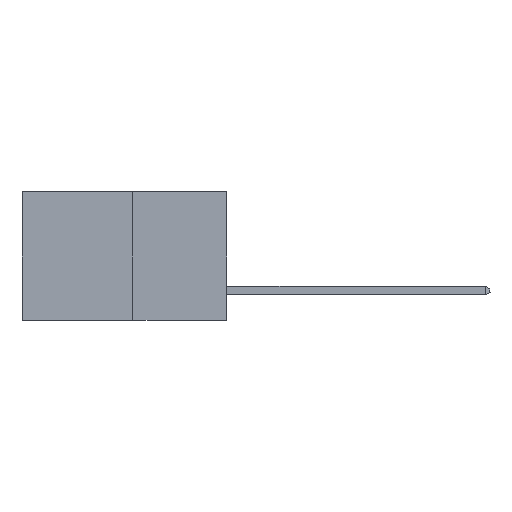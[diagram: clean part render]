
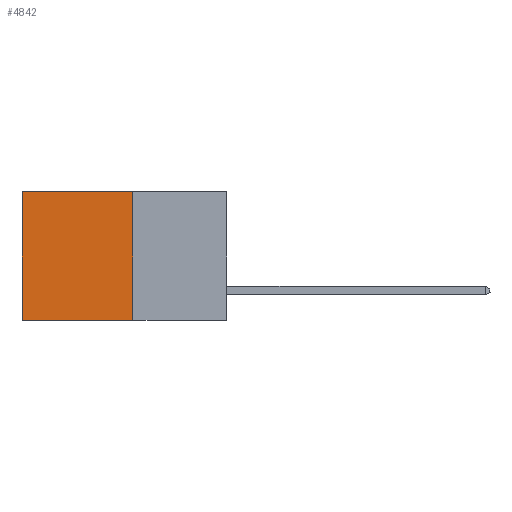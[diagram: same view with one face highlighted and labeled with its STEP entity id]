
A CAD part, left-side view. The second image highlights one B-rep face of the part: STEP entity #4842.
In plain terms, the highlighted planar face has unit normal (-1, 0, 0).
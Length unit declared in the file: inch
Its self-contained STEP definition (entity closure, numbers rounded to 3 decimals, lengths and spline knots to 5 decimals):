
#202 = CARTESIAN_POINT ( 'NONE',  ( 0.277, 0.27, -0.37 ) ) ;
#828 = ORIENTED_EDGE ( 'NONE', *, *, #5445, .F. ) ;
#1457 = DIRECTION ( 'NONE',  ( 1., 0., 0. ) ) ;
#1484 = LINE ( 'NONE', #5048, #11333 ) ;
#2099 = CARTESIAN_POINT ( 'NONE',  ( 0.277, 0.59, -0.37 ) ) ;
#2106 = DIRECTION ( 'NONE',  ( 0., 0., -1. ) ) ;
#2250 = VECTOR ( 'NONE', #4438, 39.37008 ) ;
#2484 = LINE ( 'NONE', #3314, #5390 ) ;
#3227 = VERTEX_POINT ( 'NONE', #12130 ) ;
#3314 = CARTESIAN_POINT ( 'NONE',  ( 0.277, 0.59, -0.37 ) ) ;
#3928 = PLANE ( 'NONE',  #4241 ) ;
#4241 = AXIS2_PLACEMENT_3D ( 'NONE', #202, #1457, #10121 ) ;
#4355 = DIRECTION ( 'NONE',  ( 0., 1., 0. ) ) ;
#4438 = DIRECTION ( 'NONE',  ( 0., 1., 0. ) ) ;
#4552 = EDGE_LOOP ( 'NONE', ( #14120, #14509, #828, #4939 ) ) ;
#4842 = ADVANCED_FACE ( 'NONE', ( #13642 ), #3928, .F. ) ;
#4939 = ORIENTED_EDGE ( 'NONE', *, *, #13755, .T. ) ;
#5048 = CARTESIAN_POINT ( 'NONE',  ( 0.277, 0.27, -0.37 ) ) ;
#5160 = VERTEX_POINT ( 'NONE', #8187 ) ;
#5191 = EDGE_CURVE ( 'NONE', #5160, #11857, #2484, .T. ) ;
#5390 = VECTOR ( 'NONE', #2106, 39.37008 ) ;
#5445 = EDGE_CURVE ( 'NONE', #3227, #8069, #1484, .T. ) ;
#6210 = CARTESIAN_POINT ( 'NONE',  ( 0.277, 0.27, -0.37 ) ) ;
#8031 = CARTESIAN_POINT ( 'NONE',  ( 0.277, 0.27, -0.37 ) ) ;
#8069 = VERTEX_POINT ( 'NONE', #6210 ) ;
#8187 = CARTESIAN_POINT ( 'NONE',  ( 0.277, 0.59, 0. ) ) ;
#10121 = DIRECTION ( 'NONE',  ( 0., 0., -1. ) ) ;
#11333 = VECTOR ( 'NONE', #14856, 39.37008 ) ;
#11810 = CARTESIAN_POINT ( 'NONE',  ( 0.277, 0.27, 0. ) ) ;
#11857 = VERTEX_POINT ( 'NONE', #2099 ) ;
#12130 = CARTESIAN_POINT ( 'NONE',  ( 0.277, 0.27, 0. ) ) ;
#13642 = FACE_OUTER_BOUND ( 'NONE', #4552, .T. ) ;
#13755 = EDGE_CURVE ( 'NONE', #3227, #5160, #14953, .T. ) ;
#14120 = ORIENTED_EDGE ( 'NONE', *, *, #5191, .T. ) ;
#14509 = ORIENTED_EDGE ( 'NONE', *, *, #14955, .F. ) ;
#14856 = DIRECTION ( 'NONE',  ( 0., 0., -1. ) ) ;
#14953 = LINE ( 'NONE', #11810, #2250 ) ;
#14955 = EDGE_CURVE ( 'NONE', #8069, #11857, #15894, .T. ) ;
#15506 = VECTOR ( 'NONE', #4355, 39.37008 ) ;
#15894 = LINE ( 'NONE', #8031, #15506 ) ;
